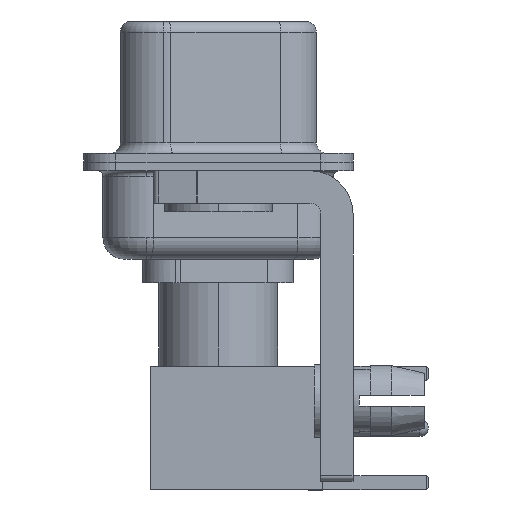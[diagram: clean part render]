
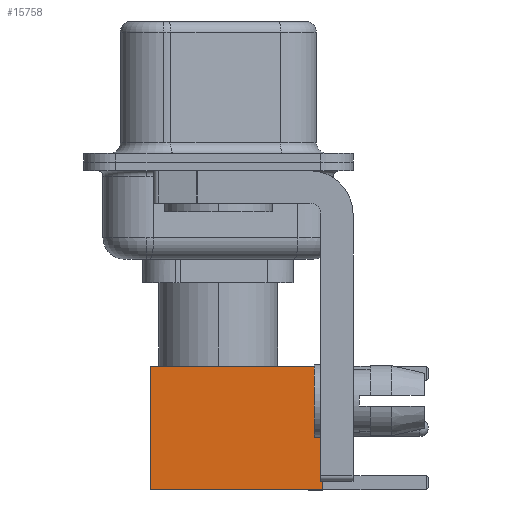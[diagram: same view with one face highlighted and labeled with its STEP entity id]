
A CAD part, left-side view. The second image highlights one B-rep face of the part: STEP entity #15758.
In plain terms, the highlighted face is planar.
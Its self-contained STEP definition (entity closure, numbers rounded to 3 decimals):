
#2024 = CARTESIAN_POINT ( 'NONE',  ( 0., 2.875, 8. ) ) ;
#2358 = DIRECTION ( 'NONE',  ( -1., 0., 0. ) ) ;
#3764 = ORIENTED_EDGE ( 'NONE', *, *, #16934, .F. ) ;
#4067 = AXIS2_PLACEMENT_3D ( 'NONE', #16774, #20408, #10001 ) ;
#4596 = VERTEX_POINT ( 'NONE', #16056 ) ;
#4894 = LINE ( 'NONE', #8151, #14721 ) ;
#4957 = FACE_OUTER_BOUND ( 'NONE', #19028, .T. ) ;
#5837 = EDGE_CURVE ( 'NONE', #10203, #6808, #4894, .T. ) ;
#6413 = CARTESIAN_POINT ( 'NONE',  ( -2.875, 2.875, 8. ) ) ;
#6808 = VERTEX_POINT ( 'NONE', #21634 ) ;
#6838 = VERTEX_POINT ( 'NONE', #6413 ) ;
#7797 = VECTOR ( 'NONE', #21251, 1000. ) ;
#8151 = CARTESIAN_POINT ( 'NONE',  ( 2.875, 2.875, 0. ) ) ;
#8259 = DIRECTION ( 'NONE',  ( 0., 0., -1. ) ) ;
#10001 = DIRECTION ( 'NONE',  ( 0., 0., 1. ) ) ;
#10203 = VERTEX_POINT ( 'NONE', #18316 ) ;
#11769 = EDGE_CURVE ( 'NONE', #6838, #4596, #13053, .T. ) ;
#12208 = PLANE ( 'NONE',  #4067 ) ;
#12460 = DIRECTION ( 'NONE',  ( -1., 0., 0. ) ) ;
#12755 = LINE ( 'NONE', #2024, #21992 ) ;
#13053 = LINE ( 'NONE', #16164, #7797 ) ;
#14087 = VECTOR ( 'NONE', #12460, 1000. ) ;
#14135 = LINE ( 'NONE', #15918, #14087 ) ;
#14721 = VECTOR ( 'NONE', #8259, 1000. ) ;
#15142 = ORIENTED_EDGE ( 'NONE', *, *, #11769, .F. ) ;
#15758 = ADVANCED_FACE ( 'NONE', ( #4957 ), #12208, .T. ) ;
#15918 = CARTESIAN_POINT ( 'NONE',  ( 0., 2.875, 0. ) ) ;
#16056 = CARTESIAN_POINT ( 'NONE',  ( -2.875, 2.875, 0. ) ) ;
#16164 = CARTESIAN_POINT ( 'NONE',  ( -2.875, 2.875, 0. ) ) ;
#16298 = EDGE_CURVE ( 'NONE', #6808, #4596, #14135, .T. ) ;
#16774 = CARTESIAN_POINT ( 'NONE',  ( 2.875, 2.875, 0. ) ) ;
#16934 = EDGE_CURVE ( 'NONE', #10203, #6838, #12755, .T. ) ;
#17565 = ORIENTED_EDGE ( 'NONE', *, *, #5837, .T. ) ;
#18316 = CARTESIAN_POINT ( 'NONE',  ( 2.875, 2.875, 8. ) ) ;
#19028 = EDGE_LOOP ( 'NONE', ( #17565, #21651, #15142, #3764 ) ) ;
#20408 = DIRECTION ( 'NONE',  ( 0., 1., 0. ) ) ;
#21251 = DIRECTION ( 'NONE',  ( 0., 0., -1. ) ) ;
#21634 = CARTESIAN_POINT ( 'NONE',  ( 2.875, 2.875, 0. ) ) ;
#21651 = ORIENTED_EDGE ( 'NONE', *, *, #16298, .T. ) ;
#21992 = VECTOR ( 'NONE', #2358, 1000. ) ;
